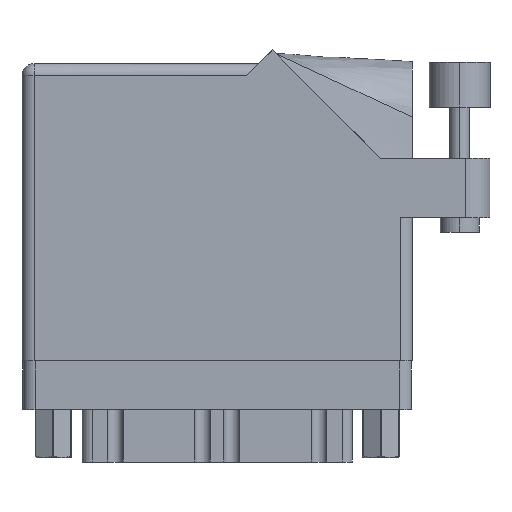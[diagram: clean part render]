
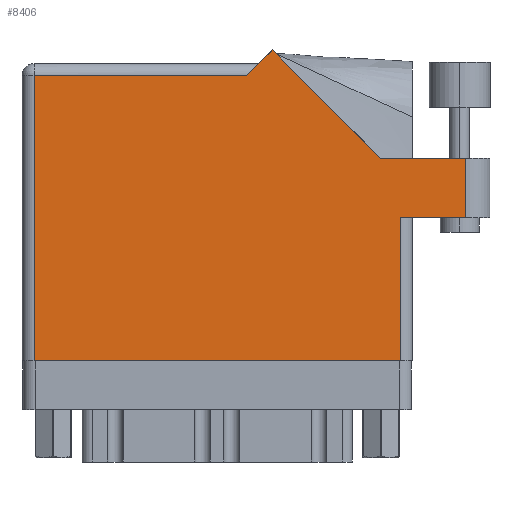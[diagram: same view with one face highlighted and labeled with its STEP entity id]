
A CAD part, front view. The second image highlights one B-rep face of the part: STEP entity #8406.
In plain terms, the highlighted face is planar.
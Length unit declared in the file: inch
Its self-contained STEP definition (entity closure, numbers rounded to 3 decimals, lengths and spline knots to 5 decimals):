
#659 = VECTOR ( 'NONE', #25680, 39.37008 ) ;
#1319 = VECTOR ( 'NONE', #32266, 39.37008 ) ;
#2229 = VERTEX_POINT ( 'NONE', #47172 ) ;
#2771 = PLANE ( 'NONE',  #15462 ) ;
#2861 = VECTOR ( 'NONE', #20859, 39.37008 ) ;
#5448 = LINE ( 'NONE', #34802, #34664 ) ;
#5985 = VERTEX_POINT ( 'NONE', #27499 ) ;
#7492 = CARTESIAN_POINT ( 'NONE',  ( 1.28771, 1.60071, 0. ) ) ;
#8294 = EDGE_CURVE ( 'NONE', #2229, #14940, #5448, .T. ) ;
#8352 = CARTESIAN_POINT ( 'NONE',  ( 1.948, 0., 0. ) ) ;
#8406 = ADVANCED_FACE ( 'NONE', ( #39140 ), #2771, .F. ) ;
#8808 = VERTEX_POINT ( 'NONE', #19348 ) ;
#9166 = ORIENTED_EDGE ( 'NONE', *, *, #19552, .T. ) ;
#9750 = DIRECTION ( 'NONE',  ( 0., 0., -1. ) ) ;
#10757 = DIRECTION ( 'NONE',  ( 1., 0., 0. ) ) ;
#11219 = CARTESIAN_POINT ( 'NONE',  ( 1.84442, 1.044, 0. ) ) ;
#12740 = EDGE_CURVE ( 'NONE', #40655, #17219, #28814, .T. ) ;
#13021 = ORIENTED_EDGE ( 'NONE', *, *, #12740, .T. ) ;
#14055 = VECTOR ( 'NONE', #27998, 39.37008 ) ;
#14181 = CARTESIAN_POINT ( 'NONE',  ( 2.41, 1.044, 0. ) ) ;
#14940 = VERTEX_POINT ( 'NONE', #40199 ) ;
#15213 = EDGE_CURVE ( 'NONE', #19976, #5985, #24598, .T. ) ;
#15462 = AXIS2_PLACEMENT_3D ( 'NONE', #47060, #9750, #42979 ) ;
#15541 = ORIENTED_EDGE ( 'NONE', *, *, #15213, .T. ) ;
#15902 = EDGE_CURVE ( 'NONE', #5985, #2229, #36530, .T. ) ;
#16512 = DIRECTION ( 'NONE',  ( 0., -1., 0. ) ) ;
#16611 = ORIENTED_EDGE ( 'NONE', *, *, #25479, .T. ) ;
#17219 = VERTEX_POINT ( 'NONE', #33487 ) ;
#17830 = CARTESIAN_POINT ( 'NONE',  ( 2.01, 0.737, 0. ) ) ;
#17893 = LINE ( 'NONE', #28945, #14055 ) ;
#18221 = CARTESIAN_POINT ( 'NONE',  ( 1.948, 0.737, 0. ) ) ;
#19287 = VERTEX_POINT ( 'NONE', #23741 ) ;
#19348 = CARTESIAN_POINT ( 'NONE',  ( 2.285, 1.044, 0. ) ) ;
#19552 = EDGE_CURVE ( 'NONE', #19287, #8808, #47564, .T. ) ;
#19976 = VERTEX_POINT ( 'NONE', #7492 ) ;
#20507 = DIRECTION ( 'NONE',  ( -0.707, -0.707, 0. ) ) ;
#20859 = DIRECTION ( 'NONE',  ( 0., 1., 0. ) ) ;
#20869 = EDGE_CURVE ( 'NONE', #14940, #40655, #40371, .T. ) ;
#23741 = CARTESIAN_POINT ( 'NONE',  ( 2.285, 0.737, 0. ) ) ;
#24085 = VECTOR ( 'NONE', #47350, 39.37008 ) ;
#24598 = LINE ( 'NONE', #39066, #24851 ) ;
#24851 = VECTOR ( 'NONE', #20507, 39.37008 ) ;
#25386 = ORIENTED_EDGE ( 'NONE', *, *, #8294, .T. ) ;
#25479 = EDGE_CURVE ( 'NONE', #43842, #19976, #17893, .T. ) ;
#25562 = VECTOR ( 'NONE', #46667, 39.37008 ) ;
#25680 = DIRECTION ( 'NONE',  ( 0., 1., 0. ) ) ;
#27322 = EDGE_CURVE ( 'NONE', #8808, #43842, #28127, .T. ) ;
#27438 = EDGE_LOOP ( 'NONE', ( #29546, #9166, #35812, #16611, #15541, #43762, #25386, #39634, #13021 ) ) ;
#27499 = CARTESIAN_POINT ( 'NONE',  ( 1.155, 1.468, 0. ) ) ;
#27998 = DIRECTION ( 'NONE',  ( -0.707, 0.707, 0. ) ) ;
#28127 = LINE ( 'NONE', #14181, #25562 ) ;
#28814 = LINE ( 'NONE', #18221, #659 ) ;
#28945 = CARTESIAN_POINT ( 'NONE',  ( 1.84442, 1.044, 0. ) ) ;
#29546 = ORIENTED_EDGE ( 'NONE', *, *, #32847, .T. ) ;
#32022 = LINE ( 'NONE', #17830, #1319 ) ;
#32266 = DIRECTION ( 'NONE',  ( 1., 0., 0. ) ) ;
#32670 = CARTESIAN_POINT ( 'NONE',  ( 0., 1.468, 0. ) ) ;
#32847 = EDGE_CURVE ( 'NONE', #17219, #19287, #32022, .T. ) ;
#33487 = CARTESIAN_POINT ( 'NONE',  ( 1.948, 0.737, 0. ) ) ;
#34664 = VECTOR ( 'NONE', #16512, 39.37008 ) ;
#34802 = CARTESIAN_POINT ( 'NONE',  ( 0.062, 0., 0. ) ) ;
#35812 = ORIENTED_EDGE ( 'NONE', *, *, #27322, .T. ) ;
#36530 = LINE ( 'NONE', #32670, #24085 ) ;
#39066 = CARTESIAN_POINT ( 'NONE',  ( 1.217, 1.53, 0. ) ) ;
#39140 = FACE_OUTER_BOUND ( 'NONE', #27438, .T. ) ;
#39634 = ORIENTED_EDGE ( 'NONE', *, *, #20869, .T. ) ;
#40199 = CARTESIAN_POINT ( 'NONE',  ( 0.062, 0., 0. ) ) ;
#40371 = LINE ( 'NONE', #43733, #45271 ) ;
#40655 = VERTEX_POINT ( 'NONE', #8352 ) ;
#42979 = DIRECTION ( 'NONE',  ( -1., 0., 0. ) ) ;
#43733 = CARTESIAN_POINT ( 'NONE',  ( 0., 0., 0. ) ) ;
#43762 = ORIENTED_EDGE ( 'NONE', *, *, #15902, .T. ) ;
#43842 = VERTEX_POINT ( 'NONE', #11219 ) ;
#43967 = CARTESIAN_POINT ( 'NONE',  ( 2.285, 1.044, 0. ) ) ;
#45271 = VECTOR ( 'NONE', #10757, 39.37008 ) ;
#46667 = DIRECTION ( 'NONE',  ( -1., 0., 0. ) ) ;
#47060 = CARTESIAN_POINT ( 'NONE',  ( 0., 1.53, 0. ) ) ;
#47172 = CARTESIAN_POINT ( 'NONE',  ( 0.062, 1.468, 0. ) ) ;
#47350 = DIRECTION ( 'NONE',  ( -1., 0., 0. ) ) ;
#47564 = LINE ( 'NONE', #43967, #2861 ) ;
